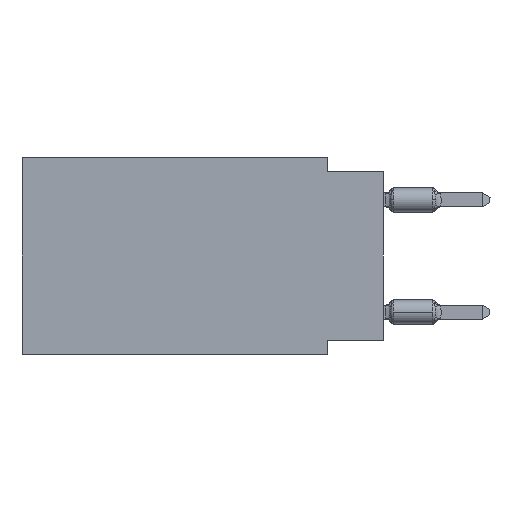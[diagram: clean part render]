
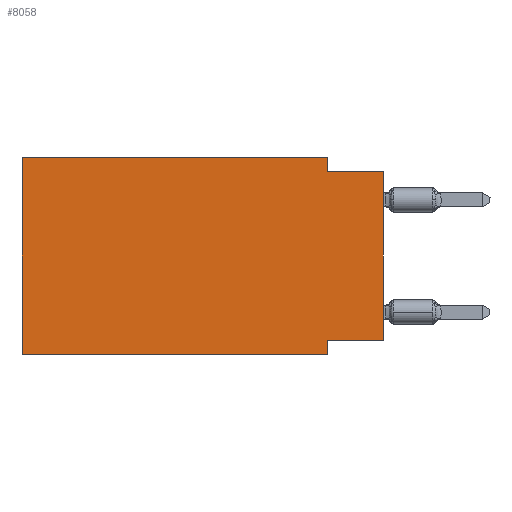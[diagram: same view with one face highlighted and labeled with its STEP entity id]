
A CAD part, left-side view. The second image highlights one B-rep face of the part: STEP entity #8058.
In plain terms, the highlighted planar face has unit normal (-1, 0, 0).
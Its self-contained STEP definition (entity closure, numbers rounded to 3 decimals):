
#383 = EDGE_CURVE ( 'NONE', #8133, #22007, #8685, .T. ) ;
#1367 = VERTEX_POINT ( 'NONE', #6991 ) ;
#1644 = ORIENTED_EDGE ( 'NONE', *, *, #2198, .F. ) ;
#2164 = VERTEX_POINT ( 'NONE', #4974 ) ;
#2198 = EDGE_CURVE ( 'NONE', #2164, #8888, #14492, .T. ) ;
#2668 = CARTESIAN_POINT ( 'NONE',  ( 0., 2.54, -8.255 ) ) ;
#3218 = DIRECTION ( 'NONE',  ( 0., 1., 0. ) ) ;
#3223 = VECTOR ( 'NONE', #7553, 1000. ) ;
#4059 = EDGE_CURVE ( 'NONE', #5698, #8133, #6682, .T. ) ;
#4974 = CARTESIAN_POINT ( 'NONE',  ( 0., 0., -8.255 ) ) ;
#5698 = VERTEX_POINT ( 'NONE', #28681 ) ;
#5703 = CARTESIAN_POINT ( 'NONE',  ( 0., 16.383, 0. ) ) ;
#5840 = EDGE_CURVE ( 'NONE', #2164, #22007, #16896, .T. ) ;
#5994 = CARTESIAN_POINT ( 'NONE',  ( 0., 2.54, -0.635 ) ) ;
#6636 = CARTESIAN_POINT ( 'NONE',  ( 0., 0., -0.635 ) ) ;
#6682 = LINE ( 'NONE', #15602, #18936 ) ;
#6953 = VECTOR ( 'NONE', #28018, 1000. ) ;
#6989 = CARTESIAN_POINT ( 'NONE',  ( 0., 0., 0. ) ) ;
#6991 = CARTESIAN_POINT ( 'NONE',  ( 0., 16.383, -8.89 ) ) ;
#7200 = ORIENTED_EDGE ( 'NONE', *, *, #28142, .F. ) ;
#7553 = DIRECTION ( 'NONE',  ( 0., 0., -1. ) ) ;
#8027 = DIRECTION ( 'NONE',  ( 0., 0., 1. ) ) ;
#8058 = ADVANCED_FACE ( 'NONE', ( #24156 ), #12588, .F. ) ;
#8133 = VERTEX_POINT ( 'NONE', #5994 ) ;
#8685 = LINE ( 'NONE', #6636, #19661 ) ;
#8732 = LINE ( 'NONE', #13404, #26109 ) ;
#8830 = VECTOR ( 'NONE', #8027, 1000. ) ;
#8888 = VERTEX_POINT ( 'NONE', #2668 ) ;
#9746 = CARTESIAN_POINT ( 'NONE',  ( 0., 2.54, -8.89 ) ) ;
#11024 = VECTOR ( 'NONE', #3218, 1000. ) ;
#11237 = AXIS2_PLACEMENT_3D ( 'NONE', #5703, #14636, #15065 ) ;
#11403 = EDGE_CURVE ( 'NONE', #8888, #28680, #20870, .T. ) ;
#12324 = ORIENTED_EDGE ( 'NONE', *, *, #22604, .T. ) ;
#12588 = PLANE ( 'NONE',  #11237 ) ;
#13404 = CARTESIAN_POINT ( 'NONE',  ( 0., 16.383, 0. ) ) ;
#13442 = CARTESIAN_POINT ( 'NONE',  ( 0., 2.54, -8.89 ) ) ;
#14333 = CARTESIAN_POINT ( 'NONE',  ( 0., 0., -8.255 ) ) ;
#14402 = DIRECTION ( 'NONE',  ( 0., 0., 1. ) ) ;
#14492 = LINE ( 'NONE', #14333, #11024 ) ;
#14636 = DIRECTION ( 'NONE',  ( 1., 0., 0. ) ) ;
#15065 = DIRECTION ( 'NONE',  ( 0., 0., -1. ) ) ;
#15556 = DIRECTION ( 'NONE',  ( 0., -1., 0. ) ) ;
#15602 = CARTESIAN_POINT ( 'NONE',  ( 0., 2.54, 0. ) ) ;
#16896 = LINE ( 'NONE', #6989, #28490 ) ;
#16962 = CARTESIAN_POINT ( 'NONE',  ( 0., 16.383, 0. ) ) ;
#17898 = ORIENTED_EDGE ( 'NONE', *, *, #21933, .F. ) ;
#18017 = ORIENTED_EDGE ( 'NONE', *, *, #383, .F. ) ;
#18270 = ORIENTED_EDGE ( 'NONE', *, *, #11403, .F. ) ;
#18936 = VECTOR ( 'NONE', #26896, 1000. ) ;
#19078 = LINE ( 'NONE', #21712, #6953 ) ;
#19661 = VECTOR ( 'NONE', #15556, 1000. ) ;
#20870 = LINE ( 'NONE', #9746, #3223 ) ;
#21581 = EDGE_LOOP ( 'NONE', ( #28371, #18017, #25071, #17898, #7200, #12324, #18270, #1644 ) ) ;
#21712 = CARTESIAN_POINT ( 'NONE',  ( 0., 16.383, -8.89 ) ) ;
#21933 = EDGE_CURVE ( 'NONE', #26736, #5698, #8732, .T. ) ;
#22007 = VERTEX_POINT ( 'NONE', #23207 ) ;
#22604 = EDGE_CURVE ( 'NONE', #1367, #28680, #19078, .T. ) ;
#23207 = CARTESIAN_POINT ( 'NONE',  ( 0., 0., -0.635 ) ) ;
#23410 = LINE ( 'NONE', #16962, #8830 ) ;
#24156 = FACE_OUTER_BOUND ( 'NONE', #21581, .T. ) ;
#24274 = DIRECTION ( 'NONE',  ( 0., -1., 0. ) ) ;
#25071 = ORIENTED_EDGE ( 'NONE', *, *, #4059, .F. ) ;
#26109 = VECTOR ( 'NONE', #24274, 1000. ) ;
#26736 = VERTEX_POINT ( 'NONE', #27999 ) ;
#26896 = DIRECTION ( 'NONE',  ( 0., 0., -1. ) ) ;
#27999 = CARTESIAN_POINT ( 'NONE',  ( 0., 16.383, 0. ) ) ;
#28018 = DIRECTION ( 'NONE',  ( 0., -1., 0. ) ) ;
#28142 = EDGE_CURVE ( 'NONE', #1367, #26736, #23410, .T. ) ;
#28371 = ORIENTED_EDGE ( 'NONE', *, *, #5840, .T. ) ;
#28490 = VECTOR ( 'NONE', #14402, 1000. ) ;
#28680 = VERTEX_POINT ( 'NONE', #13442 ) ;
#28681 = CARTESIAN_POINT ( 'NONE',  ( 0., 2.54, 0. ) ) ;
